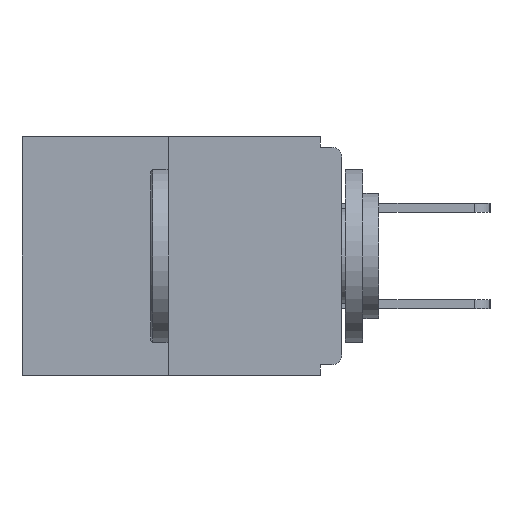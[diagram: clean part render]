
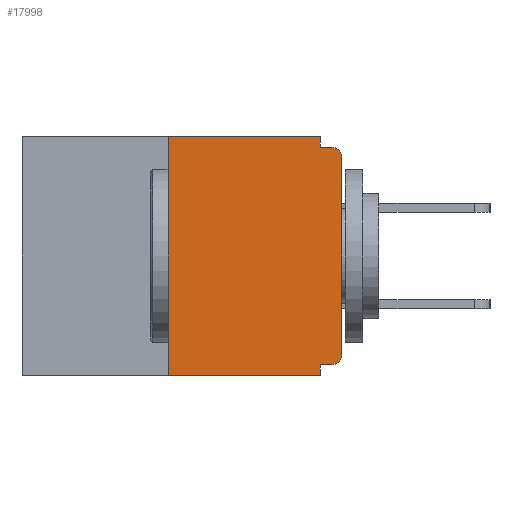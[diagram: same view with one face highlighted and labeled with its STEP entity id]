
A CAD part, left-side view. The second image highlights one B-rep face of the part: STEP entity #17998.
In plain terms, the highlighted planar face has unit normal (-1, 0, 0).
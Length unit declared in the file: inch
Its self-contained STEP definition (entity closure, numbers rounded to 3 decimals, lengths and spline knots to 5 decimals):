
#65 = LINE ( 'NONE', #10888, #15395 ) ;
#351 = CARTESIAN_POINT ( 'NONE',  ( 0., 0.015, -0.328 ) ) ;
#362 = VERTEX_POINT ( 'NONE', #18582 ) ;
#471 = DIRECTION ( 'NONE',  ( 0., -1., 0. ) ) ;
#831 = ORIENTED_EDGE ( 'NONE', *, *, #7917, .F. ) ;
#902 = EDGE_CURVE ( 'NONE', #18791, #6258, #7579, .T. ) ;
#1169 = LINE ( 'NONE', #11562, #2130 ) ;
#1368 = EDGE_CURVE ( 'NONE', #18708, #6258, #16762, .T. ) ;
#1558 = LINE ( 'NONE', #16905, #10264 ) ;
#1745 = CARTESIAN_POINT ( 'NONE',  ( 0., 0.015, -0.03 ) ) ;
#1844 = CARTESIAN_POINT ( 'NONE',  ( 0., 0.031, -0.343 ) ) ;
#2130 = VECTOR ( 'NONE', #4091, 39.37008 ) ;
#2318 = DIRECTION ( 'NONE',  ( 0., 0., -1. ) ) ;
#2512 = CARTESIAN_POINT ( 'NONE',  ( 0., 0.46, 0. ) ) ;
#3062 = CARTESIAN_POINT ( 'NONE',  ( 0., 0., -0.03 ) ) ;
#4091 = DIRECTION ( 'NONE',  ( 0., 0., 1. ) ) ;
#4135 = VERTEX_POINT ( 'NONE', #7791 ) ;
#4567 = CARTESIAN_POINT ( 'NONE',  ( 0., 0.031, 0. ) ) ;
#4808 = ORIENTED_EDGE ( 'NONE', *, *, #7533, .T. ) ;
#4810 = DIRECTION ( 'NONE',  ( 0., 1., 0. ) ) ;
#4975 = VERTEX_POINT ( 'NONE', #14714 ) ;
#5146 = CARTESIAN_POINT ( 'NONE',  ( 0., 0., -0.015 ) ) ;
#5220 = ORIENTED_EDGE ( 'NONE', *, *, #12095, .F. ) ;
#5710 = EDGE_CURVE ( 'NONE', #362, #18708, #1169, .T. ) ;
#6258 = VERTEX_POINT ( 'NONE', #14459 ) ;
#6268 = VECTOR ( 'NONE', #471, 39.37008 ) ;
#6792 = CARTESIAN_POINT ( 'NONE',  ( 0., 0.015, -0.313 ) ) ;
#6847 = DIRECTION ( 'NONE',  ( 0., 0., -1. ) ) ;
#6921 = DIRECTION ( 'NONE',  ( 1., 0., 0. ) ) ;
#6973 = ORIENTED_EDGE ( 'NONE', *, *, #5710, .T. ) ;
#7250 = DIRECTION ( 'NONE',  ( 0., 0., -1. ) ) ;
#7533 = EDGE_CURVE ( 'NONE', #10836, #362, #10048, .T. ) ;
#7579 = LINE ( 'NONE', #5146, #11799 ) ;
#7685 = VECTOR ( 'NONE', #10119, 39.37008 ) ;
#7791 = CARTESIAN_POINT ( 'NONE',  ( 0., 0.031, 0. ) ) ;
#7804 = ORIENTED_EDGE ( 'NONE', *, *, #17156, .T. ) ;
#7917 = EDGE_CURVE ( 'NONE', #10836, #17730, #1558, .T. ) ;
#7933 = CARTESIAN_POINT ( 'NONE',  ( 0., 0.46, -0.343 ) ) ;
#8054 = LINE ( 'NONE', #1844, #16320 ) ;
#8234 = DIRECTION ( 'NONE',  ( 0., 0., -1. ) ) ;
#8423 = ORIENTED_EDGE ( 'NONE', *, *, #12825, .F. ) ;
#8732 = VECTOR ( 'NONE', #7250, 39.37008 ) ;
#9392 = DIRECTION ( 'NONE',  ( 0., -1., 0. ) ) ;
#9448 = EDGE_CURVE ( 'NONE', #11005, #18683, #9546, .T. ) ;
#9546 = LINE ( 'NONE', #17594, #7685 ) ;
#10048 = CIRCLE ( 'NONE', #17082, 0.015 ) ;
#10119 = DIRECTION ( 'NONE',  ( 0., 0., 1. ) ) ;
#10264 = VECTOR ( 'NONE', #4810, 39.37008 ) ;
#10836 = VERTEX_POINT ( 'NONE', #351 ) ;
#10888 = CARTESIAN_POINT ( 'NONE',  ( 0., 0.46, 0. ) ) ;
#11005 = VERTEX_POINT ( 'NONE', #16094 ) ;
#11299 = DIRECTION ( 'NONE',  ( -1., 0., 0. ) ) ;
#11562 = CARTESIAN_POINT ( 'NONE',  ( 0., 0., 0. ) ) ;
#11799 = VECTOR ( 'NONE', #17192, 39.37008 ) ;
#12095 = EDGE_CURVE ( 'NONE', #17730, #4975, #8054, .T. ) ;
#12227 = CARTESIAN_POINT ( 'NONE',  ( 0., 0.031, -0.328 ) ) ;
#12437 = CARTESIAN_POINT ( 'NONE',  ( 0., 0.031, -0.015 ) ) ;
#12640 = AXIS2_PLACEMENT_3D ( 'NONE', #1745, #13526, #15104 ) ;
#12825 = EDGE_CURVE ( 'NONE', #4135, #18791, #15326, .T. ) ;
#13325 = ORIENTED_EDGE ( 'NONE', *, *, #1368, .T. ) ;
#13526 = DIRECTION ( 'NONE',  ( -1., 0., 0. ) ) ;
#14184 = ORIENTED_EDGE ( 'NONE', *, *, #902, .F. ) ;
#14459 = CARTESIAN_POINT ( 'NONE',  ( 0., 0.015, -0.015 ) ) ;
#14714 = CARTESIAN_POINT ( 'NONE',  ( 0., 0.031, -0.343 ) ) ;
#14948 = LINE ( 'NONE', #7933, #6268 ) ;
#15104 = DIRECTION ( 'NONE',  ( 0., 0., -1. ) ) ;
#15227 = CARTESIAN_POINT ( 'NONE',  ( 0., 0.25, 0. ) ) ;
#15326 = LINE ( 'NONE', #4567, #8732 ) ;
#15381 = ORIENTED_EDGE ( 'NONE', *, *, #18199, .F. ) ;
#15395 = VECTOR ( 'NONE', #9392, 39.37008 ) ;
#15874 = PLANE ( 'NONE',  #16853 ) ;
#15885 = FACE_OUTER_BOUND ( 'NONE', #19451, .T. ) ;
#16094 = CARTESIAN_POINT ( 'NONE',  ( 0., 0.25, -0.343 ) ) ;
#16320 = VECTOR ( 'NONE', #8234, 39.37008 ) ;
#16762 = CIRCLE ( 'NONE', #12640, 0.015 ) ;
#16853 = AXIS2_PLACEMENT_3D ( 'NONE', #2512, #6921, #6847 ) ;
#16905 = CARTESIAN_POINT ( 'NONE',  ( 0., 0., -0.328 ) ) ;
#17082 = AXIS2_PLACEMENT_3D ( 'NONE', #6792, #11299, #2318 ) ;
#17086 = ORIENTED_EDGE ( 'NONE', *, *, #9448, .F. ) ;
#17156 = EDGE_CURVE ( 'NONE', #11005, #4975, #14948, .T. ) ;
#17192 = DIRECTION ( 'NONE',  ( 0., -1., 0. ) ) ;
#17594 = CARTESIAN_POINT ( 'NONE',  ( 0., 0.25, 0. ) ) ;
#17730 = VERTEX_POINT ( 'NONE', #12227 ) ;
#17998 = ADVANCED_FACE ( 'NONE', ( #15885 ), #15874, .F. ) ;
#18199 = EDGE_CURVE ( 'NONE', #18683, #4135, #65, .T. ) ;
#18582 = CARTESIAN_POINT ( 'NONE',  ( 0., 0., -0.313 ) ) ;
#18683 = VERTEX_POINT ( 'NONE', #15227 ) ;
#18708 = VERTEX_POINT ( 'NONE', #3062 ) ;
#18791 = VERTEX_POINT ( 'NONE', #12437 ) ;
#19451 = EDGE_LOOP ( 'NONE', ( #15381, #17086, #7804, #5220, #831, #4808, #6973, #13325, #14184, #8423 ) ) ;
